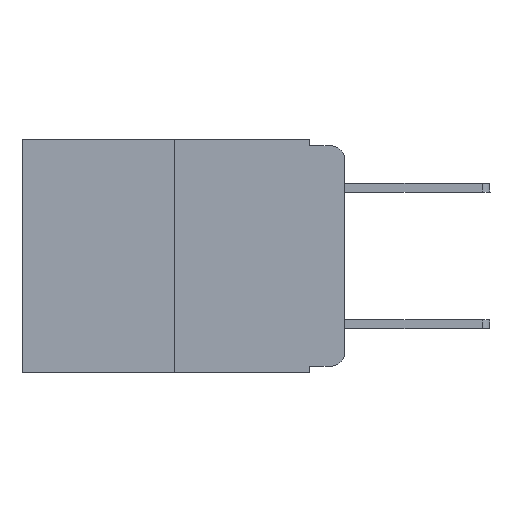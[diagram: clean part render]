
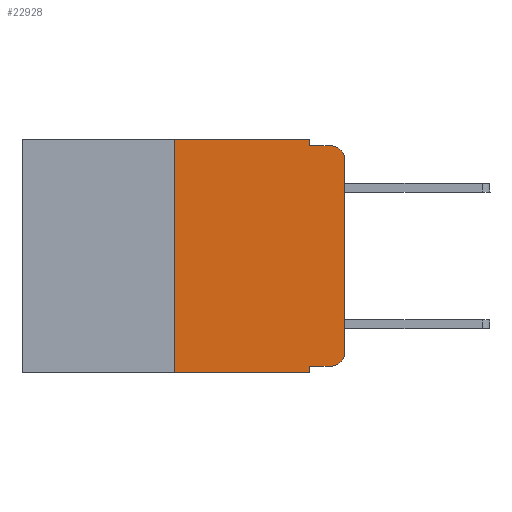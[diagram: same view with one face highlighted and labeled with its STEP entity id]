
A CAD part, left-side view. The second image highlights one B-rep face of the part: STEP entity #22928.
In plain terms, the highlighted planar face has unit normal (-1, 0, 0).
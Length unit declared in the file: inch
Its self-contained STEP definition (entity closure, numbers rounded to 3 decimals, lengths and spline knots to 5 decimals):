
#222 = CARTESIAN_POINT ( 'NONE',  ( 0., 0.473, 0. ) ) ;
#234 = DIRECTION ( 'NONE',  ( -1., 0., 0. ) ) ;
#1107 = EDGE_CURVE ( 'NONE', #3295, #18555, #17045, .T. ) ;
#1471 = VERTEX_POINT ( 'NONE', #4241 ) ;
#1661 = VERTEX_POINT ( 'NONE', #8738 ) ;
#1841 = EDGE_CURVE ( 'NONE', #1471, #14081, #11545, .T. ) ;
#1947 = CARTESIAN_POINT ( 'NONE',  ( 0., 0.02, -0.333 ) ) ;
#2029 = DIRECTION ( 'NONE',  ( 1., 0., 0. ) ) ;
#2151 = FACE_OUTER_BOUND ( 'NONE', #16523, .T. ) ;
#2213 = EDGE_CURVE ( 'NONE', #19011, #4714, #19153, .T. ) ;
#2378 = VECTOR ( 'NONE', #5621, 39.37008 ) ;
#2463 = CARTESIAN_POINT ( 'NONE',  ( 0., 0.051, -0.333 ) ) ;
#2474 = EDGE_CURVE ( 'NONE', #3295, #16372, #15612, .T. ) ;
#2995 = ORIENTED_EDGE ( 'NONE', *, *, #1841, .F. ) ;
#3295 = VERTEX_POINT ( 'NONE', #2463 ) ;
#3536 = CARTESIAN_POINT ( 'NONE',  ( 0., 0.02, -0.01 ) ) ;
#4090 = EDGE_CURVE ( 'NONE', #4714, #1471, #12956, .T. ) ;
#4241 = CARTESIAN_POINT ( 'NONE',  ( 0., 0.051, -0.01 ) ) ;
#4400 = VECTOR ( 'NONE', #17730, 39.37008 ) ;
#4714 = VERTEX_POINT ( 'NONE', #15908 ) ;
#5259 = ORIENTED_EDGE ( 'NONE', *, *, #11808, .T. ) ;
#5494 = CARTESIAN_POINT ( 'NONE',  ( 0., 0.25, 0. ) ) ;
#5621 = DIRECTION ( 'NONE',  ( 0., 0., 1. ) ) ;
#5659 = LINE ( 'NONE', #18041, #13874 ) ;
#5860 = DIRECTION ( 'NONE',  ( 0., -1., 0. ) ) ;
#5911 = DIRECTION ( 'NONE',  ( 0., 0., -1. ) ) ;
#5936 = CARTESIAN_POINT ( 'NONE',  ( 0., 0.051, 0. ) ) ;
#6773 = CARTESIAN_POINT ( 'NONE',  ( 0., 0.02, -0.313 ) ) ;
#7170 = VERTEX_POINT ( 'NONE', #8289 ) ;
#7194 = ORIENTED_EDGE ( 'NONE', *, *, #2474, .T. ) ;
#7555 = ORIENTED_EDGE ( 'NONE', *, *, #17146, .F. ) ;
#7840 = CARTESIAN_POINT ( 'NONE',  ( 0., 0.051, 0. ) ) ;
#7894 = VECTOR ( 'NONE', #20749, 39.37008 ) ;
#8289 = CARTESIAN_POINT ( 'NONE',  ( 0., 0., -0.03 ) ) ;
#8325 = EDGE_CURVE ( 'NONE', #1661, #18555, #5659, .T. ) ;
#8636 = LINE ( 'NONE', #12492, #4400 ) ;
#8738 = CARTESIAN_POINT ( 'NONE',  ( 0., 0.25, -0.343 ) ) ;
#8790 = VECTOR ( 'NONE', #12853, 39.37008 ) ;
#9065 = AXIS2_PLACEMENT_3D ( 'NONE', #222, #2029, #5911 ) ;
#11545 = LINE ( 'NONE', #22476, #13798 ) ;
#11590 = CARTESIAN_POINT ( 'NONE',  ( 0., 0., -0.313 ) ) ;
#11654 = ORIENTED_EDGE ( 'NONE', *, *, #4090, .F. ) ;
#11808 = EDGE_CURVE ( 'NONE', #16372, #22958, #18999, .T. ) ;
#11838 = PLANE ( 'NONE',  #9065 ) ;
#12120 = ORIENTED_EDGE ( 'NONE', *, *, #2213, .F. ) ;
#12477 = VECTOR ( 'NONE', #13404, 39.37008 ) ;
#12492 = CARTESIAN_POINT ( 'NONE',  ( 0., 0., 0. ) ) ;
#12853 = DIRECTION ( 'NONE',  ( 0., -1., 0. ) ) ;
#12956 = LINE ( 'NONE', #5936, #7894 ) ;
#13047 = VECTOR ( 'NONE', #19521, 39.37008 ) ;
#13063 = CARTESIAN_POINT ( 'NONE',  ( 0., 0.02, -0.03 ) ) ;
#13287 = DIRECTION ( 'NONE',  ( 0., 0., -1. ) ) ;
#13404 = DIRECTION ( 'NONE',  ( 0., 0., -1. ) ) ;
#13647 = CIRCLE ( 'NONE', #20239, 0.02 ) ;
#13798 = VECTOR ( 'NONE', #5860, 39.37008 ) ;
#13874 = VECTOR ( 'NONE', #16334, 39.37008 ) ;
#14081 = VERTEX_POINT ( 'NONE', #3536 ) ;
#15612 = LINE ( 'NONE', #21453, #13047 ) ;
#15908 = CARTESIAN_POINT ( 'NONE',  ( 0., 0.051, 0. ) ) ;
#16334 = DIRECTION ( 'NONE',  ( 0., -1., 0. ) ) ;
#16372 = VERTEX_POINT ( 'NONE', #1947 ) ;
#16523 = EDGE_LOOP ( 'NONE', ( #23259, #21896, #2995, #11654, #12120, #7555, #16918, #19293, #7194, #5259 ) ) ;
#16918 = ORIENTED_EDGE ( 'NONE', *, *, #8325, .T. ) ;
#17045 = LINE ( 'NONE', #7840, #12477 ) ;
#17146 = EDGE_CURVE ( 'NONE', #1661, #19011, #23831, .T. ) ;
#17413 = CARTESIAN_POINT ( 'NONE',  ( 0., 0.25, 0. ) ) ;
#17730 = DIRECTION ( 'NONE',  ( 0., 0., 1. ) ) ;
#18031 = EDGE_CURVE ( 'NONE', #7170, #14081, #13647, .T. ) ;
#18041 = CARTESIAN_POINT ( 'NONE',  ( 0., 0.473, -0.343 ) ) ;
#18555 = VERTEX_POINT ( 'NONE', #20061 ) ;
#18999 = CIRCLE ( 'NONE', #23643, 0.02 ) ;
#19011 = VERTEX_POINT ( 'NONE', #17413 ) ;
#19153 = LINE ( 'NONE', #22546, #8790 ) ;
#19293 = ORIENTED_EDGE ( 'NONE', *, *, #1107, .F. ) ;
#19521 = DIRECTION ( 'NONE',  ( 0., -1., 0. ) ) ;
#20061 = CARTESIAN_POINT ( 'NONE',  ( 0., 0.051, -0.343 ) ) ;
#20239 = AXIS2_PLACEMENT_3D ( 'NONE', #13063, #234, #20742 ) ;
#20742 = DIRECTION ( 'NONE',  ( 0., 0., -1. ) ) ;
#20749 = DIRECTION ( 'NONE',  ( 0., 0., -1. ) ) ;
#21332 = EDGE_CURVE ( 'NONE', #22958, #7170, #8636, .T. ) ;
#21453 = CARTESIAN_POINT ( 'NONE',  ( 0., 0.051, -0.333 ) ) ;
#21815 = DIRECTION ( 'NONE',  ( -1., 0., 0. ) ) ;
#21896 = ORIENTED_EDGE ( 'NONE', *, *, #18031, .T. ) ;
#22476 = CARTESIAN_POINT ( 'NONE',  ( 0., 0.051, -0.01 ) ) ;
#22546 = CARTESIAN_POINT ( 'NONE',  ( 0., 0.473, 0. ) ) ;
#22928 = ADVANCED_FACE ( 'NONE', ( #2151 ), #11838, .F. ) ;
#22958 = VERTEX_POINT ( 'NONE', #11590 ) ;
#23259 = ORIENTED_EDGE ( 'NONE', *, *, #21332, .T. ) ;
#23643 = AXIS2_PLACEMENT_3D ( 'NONE', #6773, #21815, #13287 ) ;
#23831 = LINE ( 'NONE', #5494, #2378 ) ;
